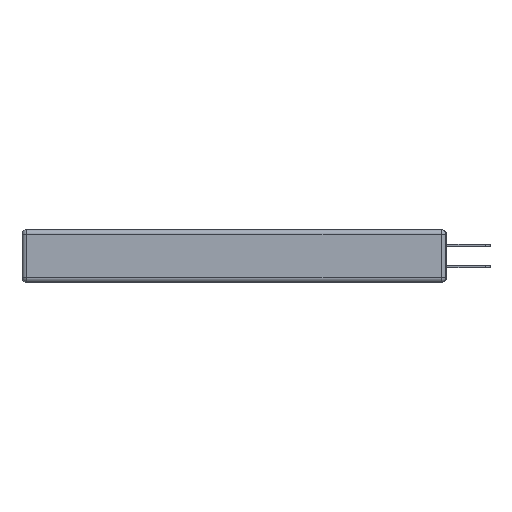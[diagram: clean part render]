
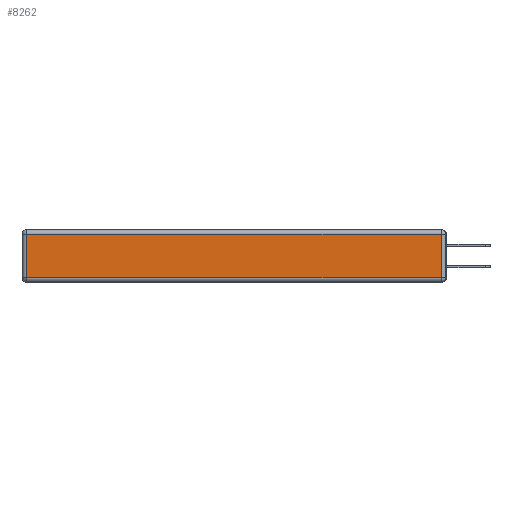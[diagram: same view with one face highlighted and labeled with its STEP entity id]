
A CAD part, left-side view. The second image highlights one B-rep face of the part: STEP entity #8262.
In plain terms, the highlighted planar face has unit normal (-1, 0, 0).
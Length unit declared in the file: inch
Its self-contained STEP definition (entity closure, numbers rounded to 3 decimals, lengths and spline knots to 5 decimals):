
#227 = VECTOR ( 'NONE', #18180, 39.37008 ) ;
#1098 = CARTESIAN_POINT ( 'NONE',  ( 0., 2.72, -0.343 ) ) ;
#2154 = VECTOR ( 'NONE', #17518, 39.37008 ) ;
#2297 = PLANE ( 'NONE',  #7030 ) ;
#2518 = LINE ( 'NONE', #1098, #227 ) ;
#2968 = ORIENTED_EDGE ( 'NONE', *, *, #5717, .T. ) ;
#3055 = VERTEX_POINT ( 'NONE', #18027 ) ;
#3466 = CARTESIAN_POINT ( 'NONE',  ( 0., 2.72, -0.313 ) ) ;
#3643 = ORIENTED_EDGE ( 'NONE', *, *, #17476, .T. ) ;
#4677 = VERTEX_POINT ( 'NONE', #3466 ) ;
#5302 = EDGE_CURVE ( 'NONE', #3055, #7983, #9446, .T. ) ;
#5717 = EDGE_CURVE ( 'NONE', #15996, #4677, #2518, .T. ) ;
#6515 = FACE_OUTER_BOUND ( 'NONE', #13424, .T. ) ;
#6578 = DIRECTION ( 'NONE',  ( -1., 0., 0. ) ) ;
#7030 = AXIS2_PLACEMENT_3D ( 'NONE', #16735, #6578, #16606 ) ;
#7100 = CARTESIAN_POINT ( 'NONE',  ( 0., 2.75, -0.03 ) ) ;
#7983 = VERTEX_POINT ( 'NONE', #12458 ) ;
#8262 = ADVANCED_FACE ( 'NONE', ( #6515 ), #2297, .T. ) ;
#9446 = LINE ( 'NONE', #14993, #17973 ) ;
#9579 = ORIENTED_EDGE ( 'NONE', *, *, #16278, .T. ) ;
#10127 = DIRECTION ( 'NONE',  ( 0., 1., 0. ) ) ;
#10368 = LINE ( 'NONE', #7100, #17756 ) ;
#10411 = LINE ( 'NONE', #13366, #2154 ) ;
#12458 = CARTESIAN_POINT ( 'NONE',  ( 0., 0.03, -0.03 ) ) ;
#13313 = CARTESIAN_POINT ( 'NONE',  ( 0., 2.72, -0.03 ) ) ;
#13366 = CARTESIAN_POINT ( 'NONE',  ( 0., 0., -0.313 ) ) ;
#13424 = EDGE_LOOP ( 'NONE', ( #9579, #15821, #3643, #2968 ) ) ;
#13430 = DIRECTION ( 'NONE',  ( 0., 0., 1. ) ) ;
#14993 = CARTESIAN_POINT ( 'NONE',  ( 0., 0.03, -0.343 ) ) ;
#15821 = ORIENTED_EDGE ( 'NONE', *, *, #5302, .T. ) ;
#15996 = VERTEX_POINT ( 'NONE', #13313 ) ;
#16278 = EDGE_CURVE ( 'NONE', #4677, #3055, #10411, .T. ) ;
#16606 = DIRECTION ( 'NONE',  ( 0., 0., 1. ) ) ;
#16735 = CARTESIAN_POINT ( 'NONE',  ( 0., 0., -0.343 ) ) ;
#17476 = EDGE_CURVE ( 'NONE', #7983, #15996, #10368, .T. ) ;
#17518 = DIRECTION ( 'NONE',  ( 0., -1., 0. ) ) ;
#17756 = VECTOR ( 'NONE', #10127, 39.37008 ) ;
#17973 = VECTOR ( 'NONE', #13430, 39.37008 ) ;
#18027 = CARTESIAN_POINT ( 'NONE',  ( 0., 0.03, -0.313 ) ) ;
#18180 = DIRECTION ( 'NONE',  ( 0., 0., -1. ) ) ;
